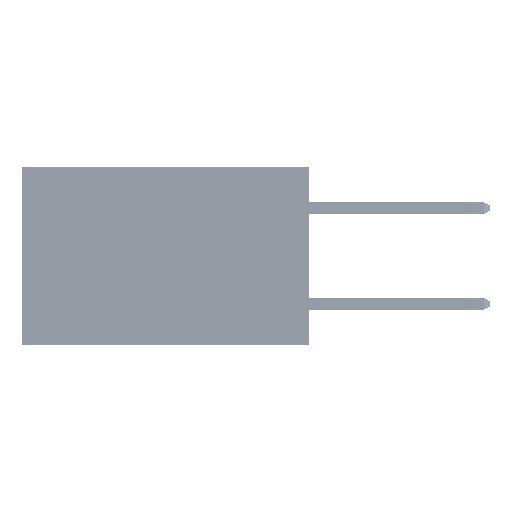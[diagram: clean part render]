
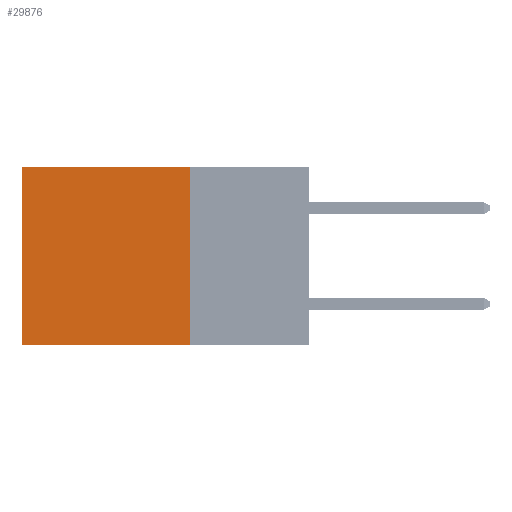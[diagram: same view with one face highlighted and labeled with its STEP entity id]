
A CAD part, left-side view. The second image highlights one B-rep face of the part: STEP entity #29876.
In plain terms, the highlighted planar face has unit normal (-1, 0, 0).
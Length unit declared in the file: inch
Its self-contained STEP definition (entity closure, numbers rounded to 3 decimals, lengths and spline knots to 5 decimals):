
#1417 = CARTESIAN_POINT ( 'NONE',  ( 0.2875, 0.25, -0.37 ) ) ;
#2249 = CARTESIAN_POINT ( 'NONE',  ( 0.2875, 0.6, -0.37 ) ) ;
#4801 = DIRECTION ( 'NONE',  ( 0., 0., -1. ) ) ;
#5030 = VECTOR ( 'NONE', #4801, 39.37008 ) ;
#6026 = FACE_OUTER_BOUND ( 'NONE', #11717, .T. ) ;
#6268 = LINE ( 'NONE', #40839, #5030 ) ;
#9226 = CARTESIAN_POINT ( 'NONE',  ( 0.2875, 0.25, 0. ) ) ;
#9735 = DIRECTION ( 'NONE',  ( 0., 1., 0. ) ) ;
#10702 = DIRECTION ( 'NONE',  ( 0., 1., 0. ) ) ;
#10920 = AXIS2_PLACEMENT_3D ( 'NONE', #50399, #14551, #18482 ) ;
#11717 = EDGE_LOOP ( 'NONE', ( #22396, #42619, #37026, #23009 ) ) ;
#14551 = DIRECTION ( 'NONE',  ( 1., 0., 0. ) ) ;
#18482 = DIRECTION ( 'NONE',  ( 0., 0., -1. ) ) ;
#21754 = CARTESIAN_POINT ( 'NONE',  ( 0.2875, 0.6, 0. ) ) ;
#22052 = CARTESIAN_POINT ( 'NONE',  ( 0.2875, 0.25, -0.37 ) ) ;
#22396 = ORIENTED_EDGE ( 'NONE', *, *, #25414, .T. ) ;
#22759 = DIRECTION ( 'NONE',  ( 0., 0., -1. ) ) ;
#23009 = ORIENTED_EDGE ( 'NONE', *, *, #26259, .T. ) ;
#23622 = VECTOR ( 'NONE', #22759, 39.37008 ) ;
#24598 = LINE ( 'NONE', #22052, #30762 ) ;
#25414 = EDGE_CURVE ( 'NONE', #28613, #36405, #6268, .T. ) ;
#26259 = EDGE_CURVE ( 'NONE', #35992, #28613, #34221, .T. ) ;
#28613 = VERTEX_POINT ( 'NONE', #21754 ) ;
#29876 = ADVANCED_FACE ( 'NONE', ( #6026 ), #49882, .F. ) ;
#30762 = VECTOR ( 'NONE', #10702, 39.37008 ) ;
#31322 = CARTESIAN_POINT ( 'NONE',  ( 0.2875, 0.25, 0. ) ) ;
#32919 = VECTOR ( 'NONE', #9735, 39.37008 ) ;
#32939 = EDGE_CURVE ( 'NONE', #38298, #36405, #24598, .T. ) ;
#33477 = CARTESIAN_POINT ( 'NONE',  ( 0.2875, 0.25, 0. ) ) ;
#34221 = LINE ( 'NONE', #33477, #32919 ) ;
#35992 = VERTEX_POINT ( 'NONE', #9226 ) ;
#36405 = VERTEX_POINT ( 'NONE', #2249 ) ;
#37026 = ORIENTED_EDGE ( 'NONE', *, *, #46177, .F. ) ;
#38298 = VERTEX_POINT ( 'NONE', #1417 ) ;
#40839 = CARTESIAN_POINT ( 'NONE',  ( 0.2875, 0.6, 0. ) ) ;
#42619 = ORIENTED_EDGE ( 'NONE', *, *, #32939, .F. ) ;
#46177 = EDGE_CURVE ( 'NONE', #35992, #38298, #47721, .T. ) ;
#47721 = LINE ( 'NONE', #31322, #23622 ) ;
#49882 = PLANE ( 'NONE',  #10920 ) ;
#50399 = CARTESIAN_POINT ( 'NONE',  ( 0.2875, 0.25, 0. ) ) ;
